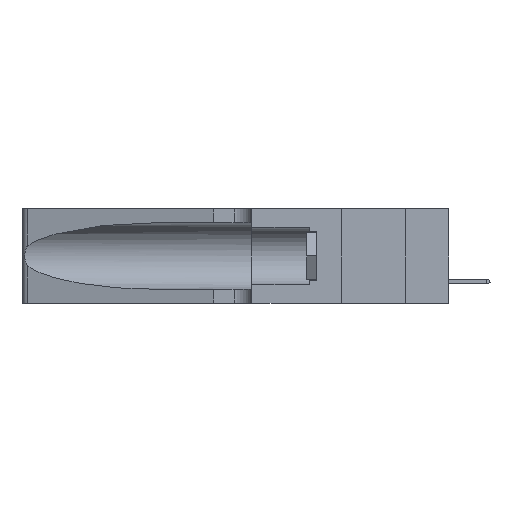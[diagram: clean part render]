
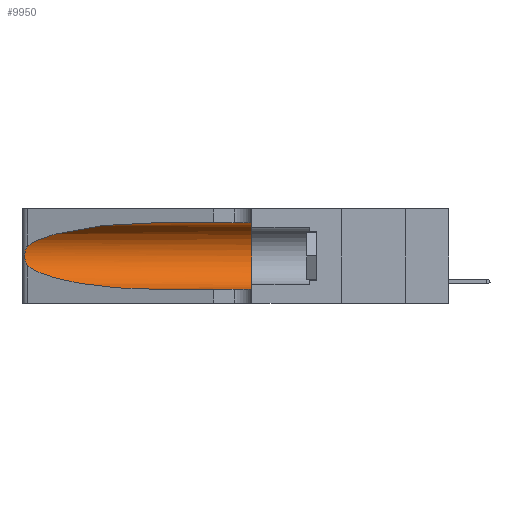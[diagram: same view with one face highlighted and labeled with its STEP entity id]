
A CAD part, left-side view. The second image highlights one B-rep face of the part: STEP entity #9950.
In plain terms, the highlighted cylindrical face has radius 3.308 mm (diameter 6.617 mm), a partial arc.
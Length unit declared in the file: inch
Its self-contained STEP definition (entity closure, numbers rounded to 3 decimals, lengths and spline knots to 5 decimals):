
#586 = CARTESIAN_POINT ( 'NONE',  ( 0.1305, 0.35, 0.185 ) ) ;
#1888 = CARTESIAN_POINT ( 'NONE',  ( 0.25487, 1.22718, 0.14631 ) ) ;
#2684 = EDGE_LOOP ( 'NONE', ( #37358, #14629, #33768, #41942, #35396, #30828 ) ) ;
#3925 = VECTOR ( 'NONE', #45434, 39.37008 ) ;
#4033 = DIRECTION ( 'NONE',  ( 0., 1., 0. ) ) ;
#5260 = CARTESIAN_POINT ( 'NONE',  ( 0.1305, 0.72297, 0.31525 ) ) ;
#5680 = AXIS2_PLACEMENT_3D ( 'NONE', #8118, #33313, #33158 ) ;
#5930 = CARTESIAN_POINT ( 'NONE',  ( 0.25487, 1.22718, 0.14631 ) ) ;
#6146 = VERTEX_POINT ( 'NONE', #16444 ) ;
#6484 = EDGE_CURVE ( 'NONE', #11316, #27574, #17904, .T. ) ;
#8118 = CARTESIAN_POINT ( 'NONE',  ( 0.1305, 1.61858, 0.185 ) ) ;
#9233 = CARTESIAN_POINT ( 'NONE',  ( 0.25555, 1.22994, 0.2215 ) ) ;
#9950 = ADVANCED_FACE ( 'NONE', ( #24598 ), #30205, .F. ) ;
#10694 = DIRECTION ( 'NONE',  ( 0., -1., 0. ) ) ;
#11316 = VERTEX_POINT ( 'NONE', #15645 ) ;
#12636 = CARTESIAN_POINT ( 'NONE',  ( 0.18966, 0.96281, 0.31525 ) ) ;
#12850 = CARTESIAN_POINT ( 'NONE',  ( 0.25787, 1.23484, 0.2124 ) ) ;
#13017 = CARTESIAN_POINT ( 'NONE',  ( 0.25639, 1.23184, 0.21858 ) ) ;
#13024 = CARTESIAN_POINT ( 'NONE',  ( 0.2373, 1.15595, 0.08982 ) ) ;
#14629 = ORIENTED_EDGE ( 'NONE', *, *, #41554, .T. ) ;
#15097 = LINE ( 'NONE', #17086, #3925 ) ;
#15645 = CARTESIAN_POINT ( 'NONE',  ( 0.1305, 0.35, 0.31525 ) ) ;
#16183 = CARTESIAN_POINT ( 'NONE',  ( 0.25487, 1.22718, 0.22369 ) ) ;
#16444 = CARTESIAN_POINT ( 'NONE',  ( 0.25487, 1.22718, 0.22369 ) ) ;
#17086 = CARTESIAN_POINT ( 'NONE',  ( 0.1305, 1.61858, 0.05475 ) ) ;
#17904 = CIRCLE ( 'NONE', #25329, 0.13025 ) ;
#22609 = EDGE_CURVE ( 'NONE', #39179, #6146, #30685, .T. ) ;
#23772 = CARTESIAN_POINT ( 'NONE',  ( 0.25856, 1.23593, 0.16098 ) ) ;
#23792 =( BOUNDED_CURVE ( )  B_SPLINE_CURVE ( 3, ( #24264, #13024, #38290, #25218 ),
 .UNSPECIFIED., .F., .F. ) 
 B_SPLINE_CURVE_WITH_KNOTS ( ( 4, 4 ),
 ( 3.44316, 4.71239 ),
 .UNSPECIFIED. ) 
 CURVE ( )  GEOMETRIC_REPRESENTATION_ITEM ( )  RATIONAL_B_SPLINE_CURVE ( ( 1., 0.87, 0.87, 1. ) ) 
 REPRESENTATION_ITEM ( '' )  );
#24264 = CARTESIAN_POINT ( 'NONE',  ( 0.25487, 1.22718, 0.14631 ) ) ;
#24598 = FACE_OUTER_BOUND ( 'NONE', #2684, .T. ) ;
#25218 = CARTESIAN_POINT ( 'NONE',  ( 0.1305, 0.72297, 0.05475 ) ) ;
#25329 = AXIS2_PLACEMENT_3D ( 'NONE', #586, #4033, #46233 ) ;
#26789 = CARTESIAN_POINT ( 'NONE',  ( 0.1305, 1.61858, 0.31525 ) ) ;
#27067 = LINE ( 'NONE', #26789, #36613 ) ;
#27197 = CARTESIAN_POINT ( 'NONE',  ( 0.26018, 1.23835, 0.19895 ) ) ;
#27574 = VERTEX_POINT ( 'NONE', #45104 ) ;
#30083 = B_SPLINE_CURVE_WITH_KNOTS ( 'NONE', 3,
 ( #30668, #9233, #13017, #12850, #38200, #27197, #37874, #30830, #41458, #23772, #30994, #41770, #45023, #5930 ),
 .UNSPECIFIED., .F., .F.,
 ( 4, 2, 2, 2, 2, 2, 4 ),
 ( 0., 0.00027, 0.00053, 0.00107, 0.0016, 0.00187, 0.00214 ),
 .UNSPECIFIED. ) ;
#30205 = CYLINDRICAL_SURFACE ( 'NONE', #5680, 0.13025 ) ;
#30668 = CARTESIAN_POINT ( 'NONE',  ( 0.25487, 1.22718, 0.22369 ) ) ;
#30685 =( BOUNDED_CURVE ( )  B_SPLINE_CURVE ( 3, ( #5260, #12636, #37690, #16183 ),
 .UNSPECIFIED., .F., .F. ) 
 B_SPLINE_CURVE_WITH_KNOTS ( ( 4, 4 ),
 ( 1.5708, 2.84003 ),
 .UNSPECIFIED. ) 
 CURVE ( )  GEOMETRIC_REPRESENTATION_ITEM ( )  RATIONAL_B_SPLINE_CURVE ( ( 1., 0.87, 0.87, 1. ) ) 
 REPRESENTATION_ITEM ( '' )  );
#30723 = EDGE_CURVE ( 'NONE', #39179, #11316, #27067, .T. ) ;
#30828 = ORIENTED_EDGE ( 'NONE', *, *, #30723, .F. ) ;
#30830 = CARTESIAN_POINT ( 'NONE',  ( 0.26075, 1.23896, 0.178 ) ) ;
#30994 = CARTESIAN_POINT ( 'NONE',  ( 0.25789, 1.23486, 0.15765 ) ) ;
#31611 = VERTEX_POINT ( 'NONE', #38394 ) ;
#33158 = DIRECTION ( 'NONE',  ( 0., 0., -1. ) ) ;
#33313 = DIRECTION ( 'NONE',  ( 0., -1., 0. ) ) ;
#33768 = ORIENTED_EDGE ( 'NONE', *, *, #39986, .T. ) ;
#35271 = VERTEX_POINT ( 'NONE', #1888 ) ;
#35302 = EDGE_CURVE ( 'NONE', #31611, #27574, #15097, .T. ) ;
#35396 = ORIENTED_EDGE ( 'NONE', *, *, #6484, .F. ) ;
#36613 = VECTOR ( 'NONE', #10694, 39.37008 ) ;
#37358 = ORIENTED_EDGE ( 'NONE', *, *, #22609, .T. ) ;
#37690 = CARTESIAN_POINT ( 'NONE',  ( 0.2373, 1.15595, 0.28018 ) ) ;
#37874 = CARTESIAN_POINT ( 'NONE',  ( 0.26075, 1.23896, 0.19203 ) ) ;
#38200 = CARTESIAN_POINT ( 'NONE',  ( 0.25854, 1.2359, 0.20912 ) ) ;
#38290 = CARTESIAN_POINT ( 'NONE',  ( 0.18966, 0.96281, 0.05475 ) ) ;
#38394 = CARTESIAN_POINT ( 'NONE',  ( 0.1305, 0.72297, 0.05475 ) ) ;
#38747 = CARTESIAN_POINT ( 'NONE',  ( 0.1305, 0.72297, 0.31525 ) ) ;
#39179 = VERTEX_POINT ( 'NONE', #38747 ) ;
#39986 = EDGE_CURVE ( 'NONE', #35271, #31611, #23792, .T. ) ;
#41458 = CARTESIAN_POINT ( 'NONE',  ( 0.26017, 1.23833, 0.17102 ) ) ;
#41554 = EDGE_CURVE ( 'NONE', #6146, #35271, #30083, .T. ) ;
#41770 = CARTESIAN_POINT ( 'NONE',  ( 0.25639, 1.23186, 0.15144 ) ) ;
#41942 = ORIENTED_EDGE ( 'NONE', *, *, #35302, .T. ) ;
#45023 = CARTESIAN_POINT ( 'NONE',  ( 0.25555, 1.22993, 0.14849 ) ) ;
#45104 = CARTESIAN_POINT ( 'NONE',  ( 0.1305, 0.35, 0.05475 ) ) ;
#45434 = DIRECTION ( 'NONE',  ( 0., -1., 0. ) ) ;
#46233 = DIRECTION ( 'NONE',  ( 0., 0., 1. ) ) ;
